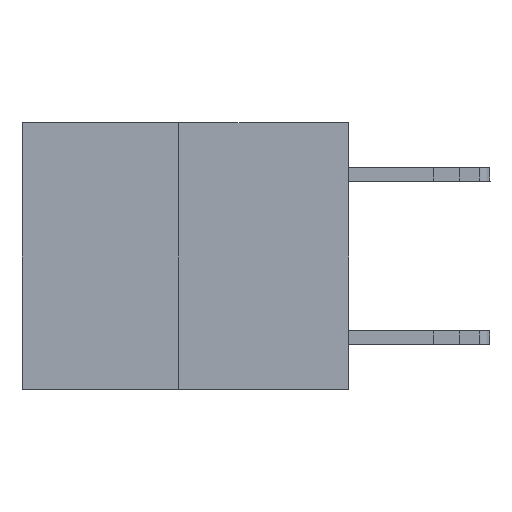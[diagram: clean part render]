
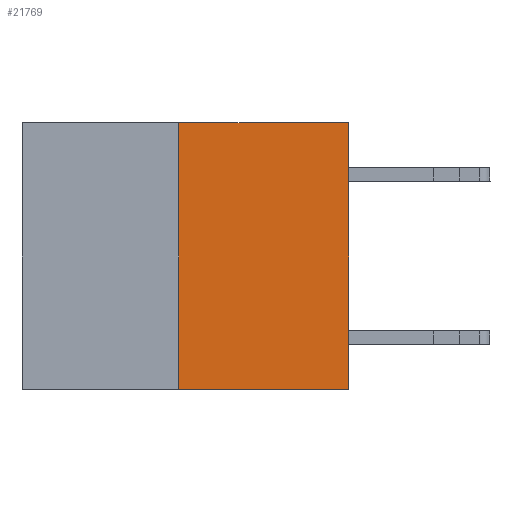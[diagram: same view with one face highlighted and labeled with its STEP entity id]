
A CAD part, left-side view. The second image highlights one B-rep face of the part: STEP entity #21769.
In plain terms, the highlighted planar face has unit normal (-1, 0, 0).
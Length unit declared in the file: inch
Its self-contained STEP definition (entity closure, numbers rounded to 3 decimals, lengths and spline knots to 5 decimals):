
#454 = DIRECTION ( 'NONE',  ( 1., 0., 0. ) ) ;
#630 = DIRECTION ( 'NONE',  ( 0., 0., 1. ) ) ;
#1313 = LINE ( 'NONE', #22657, #6043 ) ;
#2225 = CARTESIAN_POINT ( 'NONE',  ( 0., 0., 0. ) ) ;
#3261 = LINE ( 'NONE', #6506, #24061 ) ;
#4795 = VERTEX_POINT ( 'NONE', #15369 ) ;
#4870 = EDGE_CURVE ( 'NONE', #4795, #8985, #25029, .T. ) ;
#5536 = VERTEX_POINT ( 'NONE', #19614 ) ;
#5916 = ORIENTED_EDGE ( 'NONE', *, *, #21801, .F. ) ;
#6043 = VECTOR ( 'NONE', #630, 39.37008 ) ;
#6245 = VERTEX_POINT ( 'NONE', #19309 ) ;
#6328 = VECTOR ( 'NONE', #18939, 39.37008 ) ;
#6506 = CARTESIAN_POINT ( 'NONE',  ( 0., 0.6, -0.49 ) ) ;
#8553 = CARTESIAN_POINT ( 'NONE',  ( 0., 0.6, 0. ) ) ;
#8721 = PLANE ( 'NONE',  #21287 ) ;
#8985 = VERTEX_POINT ( 'NONE', #20200 ) ;
#10103 = LINE ( 'NONE', #18759, #6328 ) ;
#10754 = DIRECTION ( 'NONE',  ( 0., 0., -1. ) ) ;
#15369 = CARTESIAN_POINT ( 'NONE',  ( 0., 0., -0.49 ) ) ;
#18634 = ORIENTED_EDGE ( 'NONE', *, *, #24900, .F. ) ;
#18663 = FACE_OUTER_BOUND ( 'NONE', #20784, .T. ) ;
#18759 = CARTESIAN_POINT ( 'NONE',  ( 0., 0.6, 0. ) ) ;
#18939 = DIRECTION ( 'NONE',  ( 0., -1., 0. ) ) ;
#19309 = CARTESIAN_POINT ( 'NONE',  ( 0., 0.312, 0. ) ) ;
#19614 = CARTESIAN_POINT ( 'NONE',  ( 0., 0.312, -0.49 ) ) ;
#19654 = VECTOR ( 'NONE', #26012, 39.37008 ) ;
#20200 = CARTESIAN_POINT ( 'NONE',  ( 0., 0., 0. ) ) ;
#20384 = EDGE_CURVE ( 'NONE', #5536, #4795, #3261, .T. ) ;
#20476 = ORIENTED_EDGE ( 'NONE', *, *, #20384, .T. ) ;
#20690 = DIRECTION ( 'NONE',  ( 0., -1., 0. ) ) ;
#20784 = EDGE_LOOP ( 'NONE', ( #5916, #20476, #24013, #18634 ) ) ;
#21287 = AXIS2_PLACEMENT_3D ( 'NONE', #8553, #454, #10754 ) ;
#21769 = ADVANCED_FACE ( 'NONE', ( #18663 ), #8721, .F. ) ;
#21801 = EDGE_CURVE ( 'NONE', #5536, #6245, #1313, .T. ) ;
#22657 = CARTESIAN_POINT ( 'NONE',  ( 0., 0.312, -0.49 ) ) ;
#24013 = ORIENTED_EDGE ( 'NONE', *, *, #4870, .T. ) ;
#24061 = VECTOR ( 'NONE', #20690, 39.37008 ) ;
#24900 = EDGE_CURVE ( 'NONE', #6245, #8985, #10103, .T. ) ;
#25029 = LINE ( 'NONE', #2225, #19654 ) ;
#26012 = DIRECTION ( 'NONE',  ( 0., 0., 1. ) ) ;
